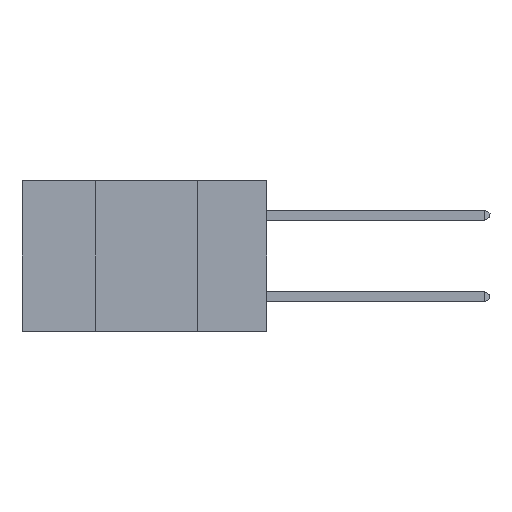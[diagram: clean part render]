
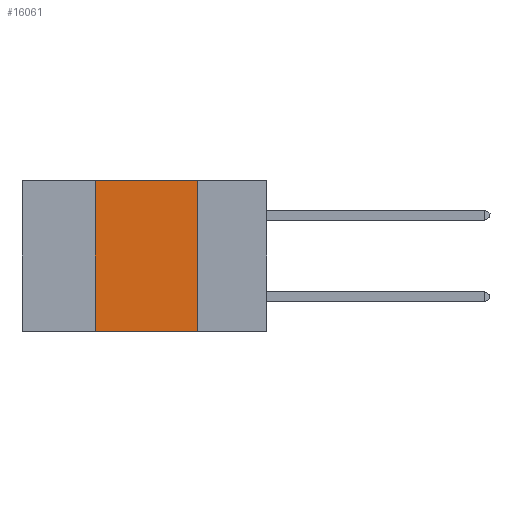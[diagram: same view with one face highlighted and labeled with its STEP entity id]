
A CAD part, left-side view. The second image highlights one B-rep face of the part: STEP entity #16061.
In plain terms, the highlighted planar face has unit normal (-1, 0, 0).
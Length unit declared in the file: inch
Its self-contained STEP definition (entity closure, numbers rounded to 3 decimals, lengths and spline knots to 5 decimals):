
#1055 = FACE_OUTER_BOUND ( 'NONE', #11338, .T. ) ;
#1222 = CARTESIAN_POINT ( 'NONE',  ( 0., 0.42, -0.37 ) ) ;
#2077 = LINE ( 'NONE', #8565, #14737 ) ;
#3630 = DIRECTION ( 'NONE',  ( 0., 0., 1. ) ) ;
#3645 = EDGE_CURVE ( 'NONE', #12409, #11536, #6554, .T. ) ;
#3821 = CARTESIAN_POINT ( 'NONE',  ( 0., 0.42, 0. ) ) ;
#4416 = ORIENTED_EDGE ( 'NONE', *, *, #12121, .F. ) ;
#4482 = LINE ( 'NONE', #10755, #11334 ) ;
#4517 = ORIENTED_EDGE ( 'NONE', *, *, #11520, .F. ) ;
#4608 = ORIENTED_EDGE ( 'NONE', *, *, #3645, .F. ) ;
#4647 = ORIENTED_EDGE ( 'NONE', *, *, #9505, .T. ) ;
#4965 = CARTESIAN_POINT ( 'NONE',  ( 0., 0.17, -0.37 ) ) ;
#6554 = LINE ( 'NONE', #3821, #9427 ) ;
#8136 = DIRECTION ( 'NONE',  ( 0., 0., -1. ) ) ;
#8403 = DIRECTION ( 'NONE',  ( 0., -1., 0. ) ) ;
#8565 = CARTESIAN_POINT ( 'NONE',  ( 0., 0.6, -0.37 ) ) ;
#9312 = PLANE ( 'NONE',  #12966 ) ;
#9427 = VECTOR ( 'NONE', #3630, 39.37008 ) ;
#9505 = EDGE_CURVE ( 'NONE', #12409, #11678, #2077, .T. ) ;
#10102 = LINE ( 'NONE', #15443, #12795 ) ;
#10755 = CARTESIAN_POINT ( 'NONE',  ( 0., 0.17, 0. ) ) ;
#11334 = VECTOR ( 'NONE', #14289, 39.37008 ) ;
#11338 = EDGE_LOOP ( 'NONE', ( #4416, #4517, #4608, #4647 ) ) ;
#11520 = EDGE_CURVE ( 'NONE', #11536, #11636, #10102, .T. ) ;
#11536 = VERTEX_POINT ( 'NONE', #11923 ) ;
#11636 = VERTEX_POINT ( 'NONE', #15704 ) ;
#11678 = VERTEX_POINT ( 'NONE', #4965 ) ;
#11923 = CARTESIAN_POINT ( 'NONE',  ( 0., 0.42, 0. ) ) ;
#12121 = EDGE_CURVE ( 'NONE', #11636, #11678, #4482, .T. ) ;
#12409 = VERTEX_POINT ( 'NONE', #1222 ) ;
#12795 = VECTOR ( 'NONE', #8403, 39.37008 ) ;
#12966 = AXIS2_PLACEMENT_3D ( 'NONE', #14000, #15240, #8136 ) ;
#13236 = DIRECTION ( 'NONE',  ( 0., -1., 0. ) ) ;
#14000 = CARTESIAN_POINT ( 'NONE',  ( 0., 0.6, 0. ) ) ;
#14289 = DIRECTION ( 'NONE',  ( 0., 0., -1. ) ) ;
#14737 = VECTOR ( 'NONE', #13236, 39.37008 ) ;
#15240 = DIRECTION ( 'NONE',  ( 1., 0., 0. ) ) ;
#15443 = CARTESIAN_POINT ( 'NONE',  ( 0., 0.6, 0. ) ) ;
#15704 = CARTESIAN_POINT ( 'NONE',  ( 0., 0.17, 0. ) ) ;
#16061 = ADVANCED_FACE ( 'NONE', ( #1055 ), #9312, .F. ) ;
